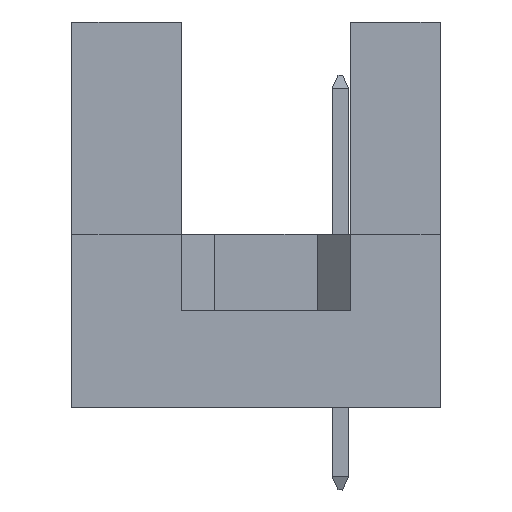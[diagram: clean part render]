
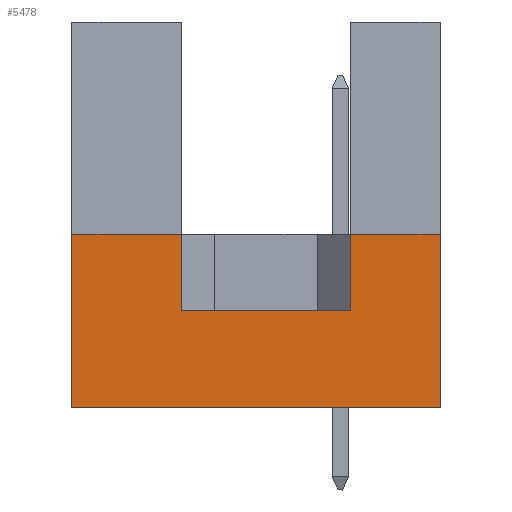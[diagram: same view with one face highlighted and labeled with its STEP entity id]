
A CAD part, left-side view. The second image highlights one B-rep face of the part: STEP entity #5478.
In plain terms, the highlighted planar face has unit normal (-1, 0, 0).
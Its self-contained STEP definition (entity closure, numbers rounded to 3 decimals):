
#22 = VECTOR ( 'NONE', #3889, 1000. ) ;
#162 = VECTOR ( 'NONE', #6196, 1000. ) ;
#277 = ORIENTED_EDGE ( 'NONE', *, *, #1173, .T. ) ;
#280 = CARTESIAN_POINT ( 'NONE',  ( -19.9, 11.1, 5.2 ) ) ;
#312 = CARTESIAN_POINT ( 'NONE',  ( -19.9, 11.1, 5.2 ) ) ;
#326 = FACE_OUTER_BOUND ( 'NONE', #405, .T. ) ;
#405 = EDGE_LOOP ( 'NONE', ( #5750, #3300, #4117, #2033, #277, #3524, #776, #3372 ) ) ;
#509 = EDGE_CURVE ( 'NONE', #4853, #1780, #1351, .T. ) ;
#776 = ORIENTED_EDGE ( 'NONE', *, *, #3030, .F. ) ;
#777 = CARTESIAN_POINT ( 'NONE',  ( -19.9, 2.71, 2.9 ) ) ;
#814 = LINE ( 'NONE', #312, #22 ) ;
#849 = DIRECTION ( 'NONE',  ( 0., 0., 1. ) ) ;
#949 = CARTESIAN_POINT ( 'NONE',  ( -19.9, 11.1, 0. ) ) ;
#1173 = EDGE_CURVE ( 'NONE', #4853, #1538, #5724, .T. ) ;
#1253 = CARTESIAN_POINT ( 'NONE',  ( -19.9, 7.79, 5.2 ) ) ;
#1337 = CARTESIAN_POINT ( 'NONE',  ( -19.9, 2.71, 5.2 ) ) ;
#1351 = LINE ( 'NONE', #3979, #4215 ) ;
#1412 = CARTESIAN_POINT ( 'NONE',  ( -19.9, 7.79, 2.9 ) ) ;
#1466 = CARTESIAN_POINT ( 'NONE',  ( -19.9, 7.79, 2.9 ) ) ;
#1538 = VERTEX_POINT ( 'NONE', #6104 ) ;
#1562 = CARTESIAN_POINT ( 'NONE',  ( -19.9, 0., 5.2 ) ) ;
#1623 = DIRECTION ( 'NONE',  ( 0., 0., 1. ) ) ;
#1780 = VERTEX_POINT ( 'NONE', #1824 ) ;
#1824 = CARTESIAN_POINT ( 'NONE',  ( -19.9, 11.1, 5.2 ) ) ;
#1832 = VERTEX_POINT ( 'NONE', #777 ) ;
#1862 = CARTESIAN_POINT ( 'NONE',  ( -19.9, 2.71, 2.9 ) ) ;
#1970 = LINE ( 'NONE', #1466, #5802 ) ;
#2016 = VECTOR ( 'NONE', #1623, 1000. ) ;
#2033 = ORIENTED_EDGE ( 'NONE', *, *, #509, .F. ) ;
#2193 = CARTESIAN_POINT ( 'NONE',  ( -19.9, 0., 0. ) ) ;
#2790 = EDGE_CURVE ( 'NONE', #4224, #1832, #1970, .T. ) ;
#2879 = LINE ( 'NONE', #1862, #3504 ) ;
#2967 = AXIS2_PLACEMENT_3D ( 'NONE', #3262, #5987, #5330 ) ;
#3030 = EDGE_CURVE ( 'NONE', #3921, #4115, #814, .T. ) ;
#3053 = LINE ( 'NONE', #1412, #3527 ) ;
#3146 = EDGE_CURVE ( 'NONE', #1780, #5085, #4909, .T. ) ;
#3262 = CARTESIAN_POINT ( 'NONE',  ( -19.9, 11.1, 0. ) ) ;
#3300 = ORIENTED_EDGE ( 'NONE', *, *, #5640, .T. ) ;
#3372 = ORIENTED_EDGE ( 'NONE', *, *, #4689, .F. ) ;
#3456 = DIRECTION ( 'NONE',  ( 0., -1., 0. ) ) ;
#3504 = VECTOR ( 'NONE', #849, 1000. ) ;
#3524 = ORIENTED_EDGE ( 'NONE', *, *, #6134, .T. ) ;
#3527 = VECTOR ( 'NONE', #6518, 1000. ) ;
#3654 = CARTESIAN_POINT ( 'NONE',  ( -19.9, 7.79, 2.9 ) ) ;
#3760 = CARTESIAN_POINT ( 'NONE',  ( -19.9, 11.1, 0. ) ) ;
#3818 = DIRECTION ( 'NONE',  ( 0., -1., 0. ) ) ;
#3889 = DIRECTION ( 'NONE',  ( 0., -1., 0. ) ) ;
#3916 = VECTOR ( 'NONE', #3818, 1000. ) ;
#3921 = VERTEX_POINT ( 'NONE', #1337 ) ;
#3979 = CARTESIAN_POINT ( 'NONE',  ( -19.9, 11.1, 0. ) ) ;
#4115 = VERTEX_POINT ( 'NONE', #1562 ) ;
#4117 = ORIENTED_EDGE ( 'NONE', *, *, #3146, .F. ) ;
#4215 = VECTOR ( 'NONE', #4420, 1000. ) ;
#4224 = VERTEX_POINT ( 'NONE', #3654 ) ;
#4420 = DIRECTION ( 'NONE',  ( 0., 0., 1. ) ) ;
#4689 = EDGE_CURVE ( 'NONE', #1832, #3921, #2879, .T. ) ;
#4826 = PLANE ( 'NONE',  #2967 ) ;
#4853 = VERTEX_POINT ( 'NONE', #949 ) ;
#4909 = LINE ( 'NONE', #280, #3916 ) ;
#5085 = VERTEX_POINT ( 'NONE', #1253 ) ;
#5206 = LINE ( 'NONE', #2193, #2016 ) ;
#5330 = DIRECTION ( 'NONE',  ( 0., 0., -1. ) ) ;
#5478 = ADVANCED_FACE ( 'NONE', ( #326 ), #4826, .F. ) ;
#5640 = EDGE_CURVE ( 'NONE', #4224, #5085, #3053, .T. ) ;
#5724 = LINE ( 'NONE', #3760, #162 ) ;
#5750 = ORIENTED_EDGE ( 'NONE', *, *, #2790, .F. ) ;
#5802 = VECTOR ( 'NONE', #3456, 1000. ) ;
#5987 = DIRECTION ( 'NONE',  ( 1., 0., 0. ) ) ;
#6104 = CARTESIAN_POINT ( 'NONE',  ( -19.9, 0., 0. ) ) ;
#6134 = EDGE_CURVE ( 'NONE', #1538, #4115, #5206, .T. ) ;
#6196 = DIRECTION ( 'NONE',  ( 0., -1., 0. ) ) ;
#6518 = DIRECTION ( 'NONE',  ( 0., 0., 1. ) ) ;
